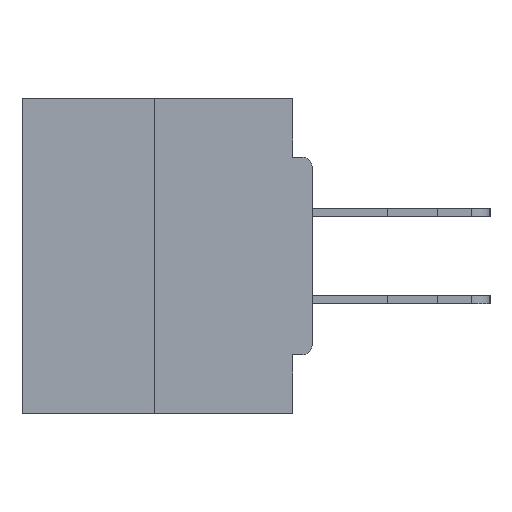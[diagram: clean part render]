
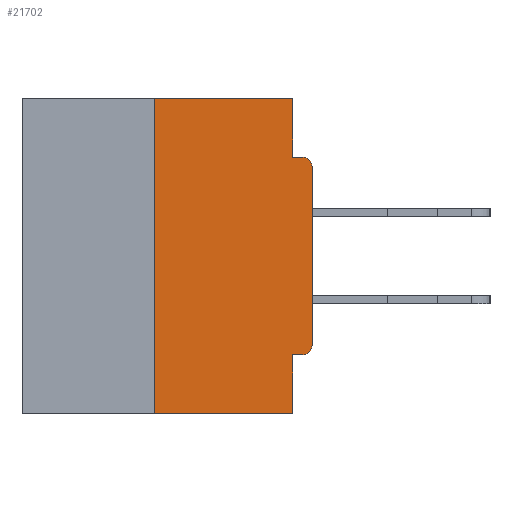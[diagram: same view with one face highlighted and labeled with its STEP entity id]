
A CAD part, left-side view. The second image highlights one B-rep face of the part: STEP entity #21702.
In plain terms, the highlighted planar face has unit normal (-1, 0, 0).
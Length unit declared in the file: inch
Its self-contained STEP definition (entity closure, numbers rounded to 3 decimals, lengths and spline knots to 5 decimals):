
#301 = VERTEX_POINT ( 'NONE', #15742 ) ;
#1439 = VECTOR ( 'NONE', #32582, 39.37008 ) ;
#2433 = EDGE_CURVE ( 'NONE', #35873, #36595, #17251, .T. ) ;
#2609 = VERTEX_POINT ( 'NONE', #41043 ) ;
#3357 = LINE ( 'NONE', #11689, #20118 ) ;
#3471 = VERTEX_POINT ( 'NONE', #28163 ) ;
#3512 = CARTESIAN_POINT ( 'NONE',  ( 0., 0., -0.4065 ) ) ;
#4503 = VECTOR ( 'NONE', #13657, 39.37008 ) ;
#4693 = ORIENTED_EDGE ( 'NONE', *, *, #30033, .T. ) ;
#4881 = DIRECTION ( 'NONE',  ( 0., 0., 1. ) ) ;
#5348 = EDGE_CURVE ( 'NONE', #301, #36120, #32098, .T. ) ;
#5455 = CARTESIAN_POINT ( 'NONE',  ( 0., 0.031, -0.5 ) ) ;
#6475 = EDGE_CURVE ( 'NONE', #36120, #2609, #39151, .T. ) ;
#6692 = VECTOR ( 'NONE', #38132, 39.37008 ) ;
#7311 = CARTESIAN_POINT ( 'NONE',  ( 0., 0., 0. ) ) ;
#8052 = CARTESIAN_POINT ( 'NONE',  ( 0., 0.25, 0. ) ) ;
#8087 = CARTESIAN_POINT ( 'NONE',  ( 0., 0.46, 0. ) ) ;
#8324 = ORIENTED_EDGE ( 'NONE', *, *, #6475, .F. ) ;
#8904 = FACE_OUTER_BOUND ( 'NONE', #12984, .T. ) ;
#9657 = CARTESIAN_POINT ( 'NONE',  ( 0., 0.031, 0. ) ) ;
#10985 = AXIS2_PLACEMENT_3D ( 'NONE', #33716, #36828, #36967 ) ;
#11515 = ORIENTED_EDGE ( 'NONE', *, *, #27757, .F. ) ;
#11689 = CARTESIAN_POINT ( 'NONE',  ( 0., 0.46, -0.5 ) ) ;
#12925 = DIRECTION ( 'NONE',  ( 0., 0., -1. ) ) ;
#12984 = EDGE_LOOP ( 'NONE', ( #36744, #11515, #4693, #14094, #26467, #23827, #19673, #27142, #8324, #38218 ) ) ;
#13657 = DIRECTION ( 'NONE',  ( 0., -1., 0. ) ) ;
#13787 = CARTESIAN_POINT ( 'NONE',  ( 0., 0.031, -0.4065 ) ) ;
#13835 = VERTEX_POINT ( 'NONE', #13787 ) ;
#14094 = ORIENTED_EDGE ( 'NONE', *, *, #14419, .F. ) ;
#14218 = VECTOR ( 'NONE', #20183, 39.37008 ) ;
#14419 = EDGE_CURVE ( 'NONE', #13835, #25546, #41218, .T. ) ;
#15287 = DIRECTION ( 'NONE',  ( 0., 0., -1. ) ) ;
#15301 = EDGE_CURVE ( 'NONE', #22109, #13835, #40107, .T. ) ;
#15742 = CARTESIAN_POINT ( 'NONE',  ( 0., 0.031, 0. ) ) ;
#16154 = EDGE_CURVE ( 'NONE', #36595, #2609, #33936, .T. ) ;
#16185 = VERTEX_POINT ( 'NONE', #8052 ) ;
#17251 = LINE ( 'NONE', #7311, #14218 ) ;
#17278 = DIRECTION ( 'NONE',  ( -1., 0., 0. ) ) ;
#17385 = AXIS2_PLACEMENT_3D ( 'NONE', #8087, #40411, #30744 ) ;
#19398 = EDGE_CURVE ( 'NONE', #22109, #35873, #38018, .T. ) ;
#19673 = ORIENTED_EDGE ( 'NONE', *, *, #2433, .T. ) ;
#20013 = CARTESIAN_POINT ( 'NONE',  ( 0., 0.031, -0.5 ) ) ;
#20118 = VECTOR ( 'NONE', #21473, 39.37008 ) ;
#20183 = DIRECTION ( 'NONE',  ( 0., 0., 1. ) ) ;
#21473 = DIRECTION ( 'NONE',  ( 0., -1., 0. ) ) ;
#21621 = CARTESIAN_POINT ( 'NONE',  ( 0., 0.25, 0. ) ) ;
#21702 = ADVANCED_FACE ( 'NONE', ( #8904 ), #40274, .F. ) ;
#22109 = VERTEX_POINT ( 'NONE', #33184 ) ;
#23827 = ORIENTED_EDGE ( 'NONE', *, *, #19398, .T. ) ;
#24403 = CARTESIAN_POINT ( 'NONE',  ( 0., 0., -0.0935 ) ) ;
#25546 = VERTEX_POINT ( 'NONE', #20013 ) ;
#26467 = ORIENTED_EDGE ( 'NONE', *, *, #15301, .F. ) ;
#26583 = CARTESIAN_POINT ( 'NONE',  ( 0., 0., -0.1085 ) ) ;
#27142 = ORIENTED_EDGE ( 'NONE', *, *, #16154, .T. ) ;
#27757 = EDGE_CURVE ( 'NONE', #3471, #16185, #39908, .T. ) ;
#27910 = LINE ( 'NONE', #29797, #4503 ) ;
#28163 = CARTESIAN_POINT ( 'NONE',  ( 0., 0.25, -0.5 ) ) ;
#28650 = VECTOR ( 'NONE', #12925, 39.37008 ) ;
#29797 = CARTESIAN_POINT ( 'NONE',  ( 0., 0.46, 0. ) ) ;
#30033 = EDGE_CURVE ( 'NONE', #3471, #25546, #3357, .T. ) ;
#30150 = CARTESIAN_POINT ( 'NONE',  ( 0., 0.015, -0.3915 ) ) ;
#30349 = AXIS2_PLACEMENT_3D ( 'NONE', #30150, #17278, #33305 ) ;
#30744 = DIRECTION ( 'NONE',  ( 0., 0., -1. ) ) ;
#31256 = VECTOR ( 'NONE', #4881, 39.37008 ) ;
#32098 = LINE ( 'NONE', #9657, #28650 ) ;
#32582 = DIRECTION ( 'NONE',  ( 0., 1., 0. ) ) ;
#32731 = CARTESIAN_POINT ( 'NONE',  ( 0., 0., -0.3915 ) ) ;
#33184 = CARTESIAN_POINT ( 'NONE',  ( 0., 0.015, -0.4065 ) ) ;
#33305 = DIRECTION ( 'NONE',  ( 0., 0., -1. ) ) ;
#33716 = CARTESIAN_POINT ( 'NONE',  ( 0., 0.015, -0.1085 ) ) ;
#33936 = CIRCLE ( 'NONE', #10985, 0.015 ) ;
#35873 = VERTEX_POINT ( 'NONE', #32731 ) ;
#36120 = VERTEX_POINT ( 'NONE', #37230 ) ;
#36591 = EDGE_CURVE ( 'NONE', #16185, #301, #27910, .T. ) ;
#36595 = VERTEX_POINT ( 'NONE', #26583 ) ;
#36744 = ORIENTED_EDGE ( 'NONE', *, *, #36591, .F. ) ;
#36828 = DIRECTION ( 'NONE',  ( -1., 0., 0. ) ) ;
#36967 = DIRECTION ( 'NONE',  ( 0., 0., -1. ) ) ;
#37230 = CARTESIAN_POINT ( 'NONE',  ( 0., 0.031, -0.0935 ) ) ;
#38018 = CIRCLE ( 'NONE', #30349, 0.015 ) ;
#38132 = DIRECTION ( 'NONE',  ( 0., -1., 0. ) ) ;
#38218 = ORIENTED_EDGE ( 'NONE', *, *, #5348, .F. ) ;
#39151 = LINE ( 'NONE', #24403, #6692 ) ;
#39908 = LINE ( 'NONE', #21621, #31256 ) ;
#40107 = LINE ( 'NONE', #3512, #1439 ) ;
#40188 = VECTOR ( 'NONE', #15287, 39.37008 ) ;
#40274 = PLANE ( 'NONE',  #17385 ) ;
#40411 = DIRECTION ( 'NONE',  ( 1., 0., 0. ) ) ;
#41043 = CARTESIAN_POINT ( 'NONE',  ( 0., 0.015, -0.0935 ) ) ;
#41218 = LINE ( 'NONE', #5455, #40188 ) ;
